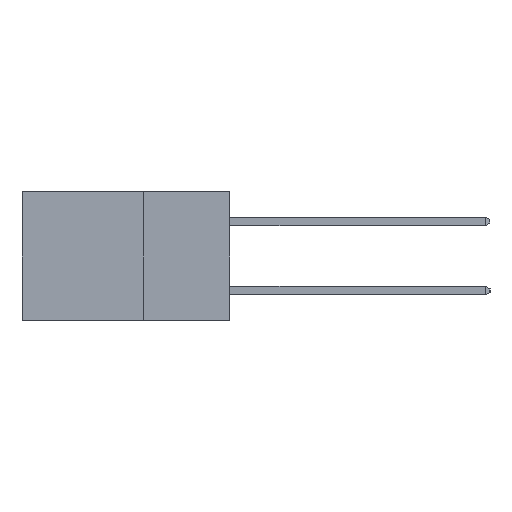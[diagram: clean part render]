
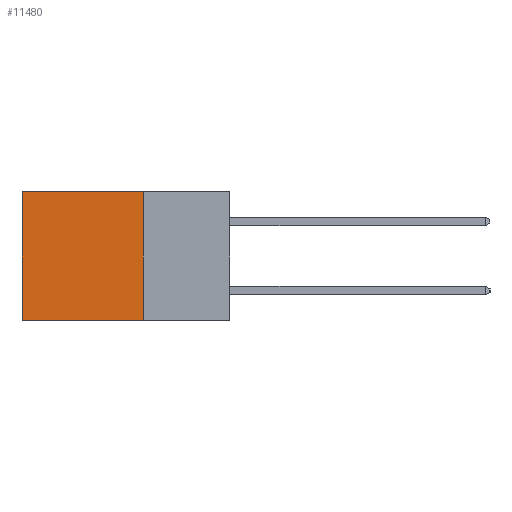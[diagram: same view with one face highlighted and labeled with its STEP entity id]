
A CAD part, left-side view. The second image highlights one B-rep face of the part: STEP entity #11480.
In plain terms, the highlighted planar face has unit normal (-1, 0, 0).
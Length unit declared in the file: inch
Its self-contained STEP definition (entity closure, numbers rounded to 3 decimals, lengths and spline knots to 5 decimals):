
#324 = CARTESIAN_POINT ( 'NONE',  ( 0.2615, 0.6, -0.37 ) ) ;
#375 = EDGE_LOOP ( 'NONE', ( #7917, #8135, #8386, #8610 ) ) ;
#610 = CARTESIAN_POINT ( 'NONE',  ( 0.2615, 0.6, 0. ) ) ;
#684 = VERTEX_POINT ( 'NONE', #2428 ) ;
#1854 = FACE_OUTER_BOUND ( 'NONE', #375, .T. ) ;
#2192 = DIRECTION ( 'NONE',  ( 0., 0., -1. ) ) ;
#2417 = LINE ( 'NONE', #13598, #5081 ) ;
#2428 = CARTESIAN_POINT ( 'NONE',  ( 0.2615, 0.25, 0. ) ) ;
#2481 = DIRECTION ( 'NONE',  ( 0., 0., -1. ) ) ;
#2580 = DIRECTION ( 'NONE',  ( 1., 0., 0. ) ) ;
#2819 = PLANE ( 'NONE',  #4309 ) ;
#2931 = CARTESIAN_POINT ( 'NONE',  ( 0.2615, 0.6, -0.37 ) ) ;
#3013 = CARTESIAN_POINT ( 'NONE',  ( 0.2615, 0.25, -0.37 ) ) ;
#3666 = VECTOR ( 'NONE', #2192, 39.37008 ) ;
#4307 = EDGE_CURVE ( 'NONE', #10614, #7995, #2417, .T. ) ;
#4309 = AXIS2_PLACEMENT_3D ( 'NONE', #3013, #2580, #2481 ) ;
#4788 = EDGE_CURVE ( 'NONE', #684, #10614, #13933, .T. ) ;
#5081 = VECTOR ( 'NONE', #13495, 39.37008 ) ;
#5411 = EDGE_CURVE ( 'NONE', #11150, #7995, #6251, .T. ) ;
#5416 = VECTOR ( 'NONE', #7458, 39.37008 ) ;
#5820 = CARTESIAN_POINT ( 'NONE',  ( 0.2615, 0.25, -0.37 ) ) ;
#6209 = DIRECTION ( 'NONE',  ( 0., 1., 0. ) ) ;
#6251 = LINE ( 'NONE', #2931, #3666 ) ;
#6350 = CARTESIAN_POINT ( 'NONE',  ( 0.2615, 0.25, 0. ) ) ;
#7413 = CARTESIAN_POINT ( 'NONE',  ( 0.2615, 0.25, -0.37 ) ) ;
#7458 = DIRECTION ( 'NONE',  ( 0., 0., -1. ) ) ;
#7917 = ORIENTED_EDGE ( 'NONE', *, *, #5411, .T. ) ;
#7995 = VERTEX_POINT ( 'NONE', #324 ) ;
#8135 = ORIENTED_EDGE ( 'NONE', *, *, #4307, .F. ) ;
#8386 = ORIENTED_EDGE ( 'NONE', *, *, #4788, .F. ) ;
#8610 = ORIENTED_EDGE ( 'NONE', *, *, #12031, .T. ) ;
#10614 = VERTEX_POINT ( 'NONE', #5820 ) ;
#11150 = VERTEX_POINT ( 'NONE', #610 ) ;
#11166 = VECTOR ( 'NONE', #6209, 39.37008 ) ;
#11480 = ADVANCED_FACE ( 'NONE', ( #1854 ), #2819, .F. ) ;
#11814 = LINE ( 'NONE', #6350, #11166 ) ;
#12031 = EDGE_CURVE ( 'NONE', #684, #11150, #11814, .T. ) ;
#13495 = DIRECTION ( 'NONE',  ( 0., 1., 0. ) ) ;
#13598 = CARTESIAN_POINT ( 'NONE',  ( 0.2615, 0.25, -0.37 ) ) ;
#13933 = LINE ( 'NONE', #7413, #5416 ) ;
